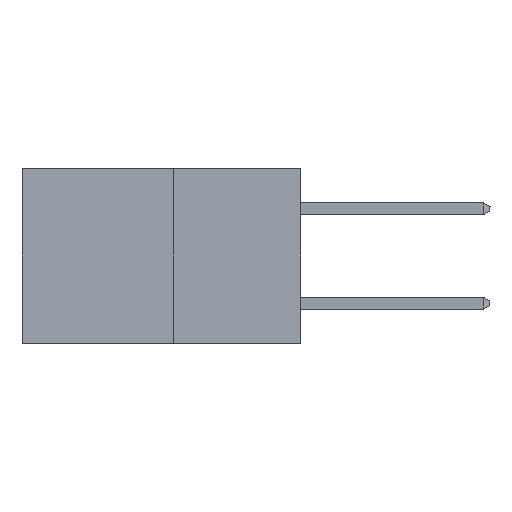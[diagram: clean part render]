
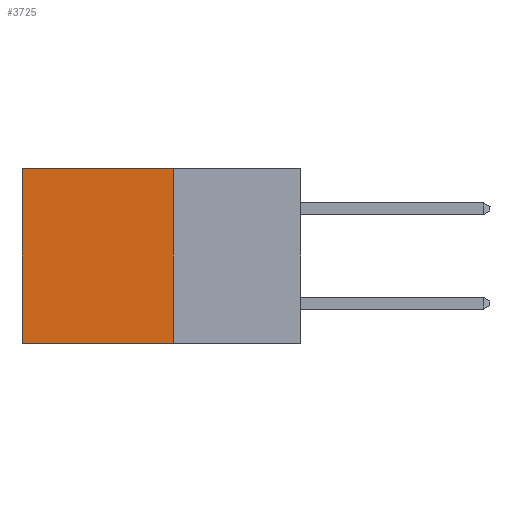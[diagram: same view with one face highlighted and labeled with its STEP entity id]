
A CAD part, left-side view. The second image highlights one B-rep face of the part: STEP entity #3725.
In plain terms, the highlighted planar face has unit normal (-1, 0, 0).
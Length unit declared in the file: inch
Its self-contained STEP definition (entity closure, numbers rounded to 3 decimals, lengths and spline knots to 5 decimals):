
#53 = VECTOR ( 'NONE', #12289, 39.37008 ) ;
#1410 = CARTESIAN_POINT ( 'NONE',  ( 0.277, 0.59, 0. ) ) ;
#1669 = CARTESIAN_POINT ( 'NONE',  ( 0.277, 0.27, -0.37 ) ) ;
#1706 = DIRECTION ( 'NONE',  ( 1., 0., 0. ) ) ;
#1724 = CARTESIAN_POINT ( 'NONE',  ( 0.277, 0.27, -0.37 ) ) ;
#1921 = EDGE_LOOP ( 'NONE', ( #10972, #11118, #11257, #12305 ) ) ;
#2350 = CARTESIAN_POINT ( 'NONE',  ( 0.277, 0.59, -0.37 ) ) ;
#2868 = DIRECTION ( 'NONE',  ( 0., 0., -1. ) ) ;
#3161 = EDGE_CURVE ( 'NONE', #3232, #9332, #8480, .T. ) ;
#3232 = VERTEX_POINT ( 'NONE', #9714 ) ;
#3383 = AXIS2_PLACEMENT_3D ( 'NONE', #1724, #1706, #3632 ) ;
#3632 = DIRECTION ( 'NONE',  ( 0., 0., -1. ) ) ;
#3725 = ADVANCED_FACE ( 'NONE', ( #7241 ), #11219, .F. ) ;
#3854 = CARTESIAN_POINT ( 'NONE',  ( 0.277, 0.27, -0.37 ) ) ;
#4836 = VECTOR ( 'NONE', #12861, 39.37008 ) ;
#5415 = VERTEX_POINT ( 'NONE', #2350 ) ;
#6419 = EDGE_CURVE ( 'NONE', #12666, #5415, #12704, .T. ) ;
#6540 = CARTESIAN_POINT ( 'NONE',  ( 0.277, 0.27, -0.37 ) ) ;
#7241 = FACE_OUTER_BOUND ( 'NONE', #1921, .T. ) ;
#7349 = LINE ( 'NONE', #3854, #12074 ) ;
#8218 = CARTESIAN_POINT ( 'NONE',  ( 0.277, 0.59, -0.37 ) ) ;
#8480 = LINE ( 'NONE', #11354, #53 ) ;
#8967 = VECTOR ( 'NONE', #2868, 39.37008 ) ;
#9332 = VERTEX_POINT ( 'NONE', #1410 ) ;
#9714 = CARTESIAN_POINT ( 'NONE',  ( 0.277, 0.27, 0. ) ) ;
#10972 = ORIENTED_EDGE ( 'NONE', *, *, #12274, .T. ) ;
#11118 = ORIENTED_EDGE ( 'NONE', *, *, #6419, .F. ) ;
#11219 = PLANE ( 'NONE',  #3383 ) ;
#11257 = ORIENTED_EDGE ( 'NONE', *, *, #12231, .F. ) ;
#11354 = CARTESIAN_POINT ( 'NONE',  ( 0.277, 0.27, 0. ) ) ;
#11784 = LINE ( 'NONE', #8218, #8967 ) ;
#12074 = VECTOR ( 'NONE', #12822, 39.37008 ) ;
#12231 = EDGE_CURVE ( 'NONE', #3232, #12666, #7349, .T. ) ;
#12274 = EDGE_CURVE ( 'NONE', #9332, #5415, #11784, .T. ) ;
#12289 = DIRECTION ( 'NONE',  ( 0., 1., 0. ) ) ;
#12305 = ORIENTED_EDGE ( 'NONE', *, *, #3161, .T. ) ;
#12666 = VERTEX_POINT ( 'NONE', #6540 ) ;
#12704 = LINE ( 'NONE', #1669, #4836 ) ;
#12822 = DIRECTION ( 'NONE',  ( 0., 0., -1. ) ) ;
#12861 = DIRECTION ( 'NONE',  ( 0., 1., 0. ) ) ;
